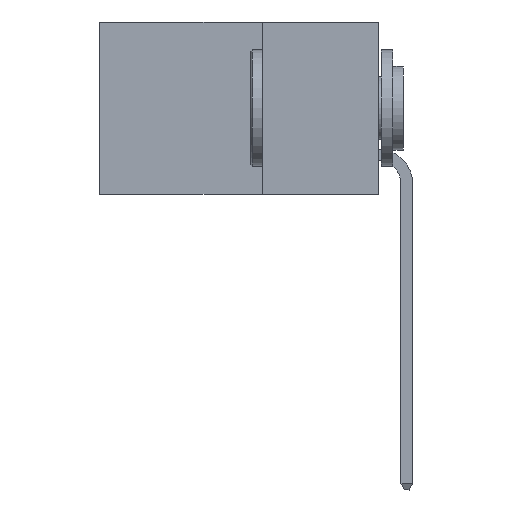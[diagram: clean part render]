
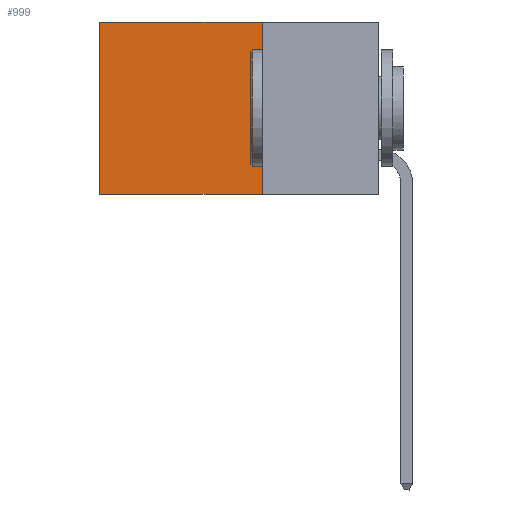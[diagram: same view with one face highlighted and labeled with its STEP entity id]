
A CAD part, left-side view. The second image highlights one B-rep face of the part: STEP entity #999.
In plain terms, the highlighted planar face has unit normal (-1, 0, 0).
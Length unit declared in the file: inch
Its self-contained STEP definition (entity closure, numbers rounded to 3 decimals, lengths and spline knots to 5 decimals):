
#75 = DIRECTION ( 'NONE',  ( 0., 0., -1. ) ) ;
#999 = ADVANCED_FACE ( 'NONE', ( #8379 ), #2125, .F. ) ;
#1003 = VERTEX_POINT ( 'NONE', #11695 ) ;
#1465 = VECTOR ( 'NONE', #16635, 39.37008 ) ;
#1682 = EDGE_CURVE ( 'NONE', #12614, #1003, #10702, .T. ) ;
#1995 = LINE ( 'NONE', #19663, #1465 ) ;
#2107 = CARTESIAN_POINT ( 'NONE',  ( 0.298, 0.25, 0. ) ) ;
#2125 = PLANE ( 'NONE',  #8407 ) ;
#2410 = VERTEX_POINT ( 'NONE', #13620 ) ;
#3619 = EDGE_CURVE ( 'NONE', #1003, #2410, #12885, .T. ) ;
#4291 = ORIENTED_EDGE ( 'NONE', *, *, #3619, .F. ) ;
#4864 = ORIENTED_EDGE ( 'NONE', *, *, #1682, .F. ) ;
#5233 = CARTESIAN_POINT ( 'NONE',  ( 0.298, 0.25, 0. ) ) ;
#5679 = CARTESIAN_POINT ( 'NONE',  ( 0.298, 0.25, -0.37 ) ) ;
#6184 = DIRECTION ( 'NONE',  ( 0., 1., 0. ) ) ;
#6451 = LINE ( 'NONE', #18887, #15054 ) ;
#8379 = FACE_OUTER_BOUND ( 'NONE', #15004, .T. ) ;
#8407 = AXIS2_PLACEMENT_3D ( 'NONE', #2107, #8659, #9409 ) ;
#8659 = DIRECTION ( 'NONE',  ( 1., 0., 0. ) ) ;
#8841 = ORIENTED_EDGE ( 'NONE', *, *, #20059, .T. ) ;
#9409 = DIRECTION ( 'NONE',  ( 0., 0., -1. ) ) ;
#9934 = ORIENTED_EDGE ( 'NONE', *, *, #16709, .T. ) ;
#10240 = VECTOR ( 'NONE', #16993, 39.37008 ) ;
#10506 = CARTESIAN_POINT ( 'NONE',  ( 0.298, 0.6, 0. ) ) ;
#10702 = LINE ( 'NONE', #5233, #10240 ) ;
#11695 = CARTESIAN_POINT ( 'NONE',  ( 0.298, 0.25, -0.37 ) ) ;
#12614 = VERTEX_POINT ( 'NONE', #20199 ) ;
#12885 = LINE ( 'NONE', #5679, #16542 ) ;
#13620 = CARTESIAN_POINT ( 'NONE',  ( 0.298, 0.6, -0.37 ) ) ;
#15004 = EDGE_LOOP ( 'NONE', ( #9934, #4291, #4864, #8841 ) ) ;
#15054 = VECTOR ( 'NONE', #75, 39.37008 ) ;
#16542 = VECTOR ( 'NONE', #6184, 39.37008 ) ;
#16635 = DIRECTION ( 'NONE',  ( 0., 1., 0. ) ) ;
#16709 = EDGE_CURVE ( 'NONE', #20100, #2410, #6451, .T. ) ;
#16993 = DIRECTION ( 'NONE',  ( 0., 0., -1. ) ) ;
#18887 = CARTESIAN_POINT ( 'NONE',  ( 0.298, 0.6, 0. ) ) ;
#19663 = CARTESIAN_POINT ( 'NONE',  ( 0.298, 0.25, 0. ) ) ;
#20059 = EDGE_CURVE ( 'NONE', #12614, #20100, #1995, .T. ) ;
#20100 = VERTEX_POINT ( 'NONE', #10506 ) ;
#20199 = CARTESIAN_POINT ( 'NONE',  ( 0.298, 0.25, 0. ) ) ;
